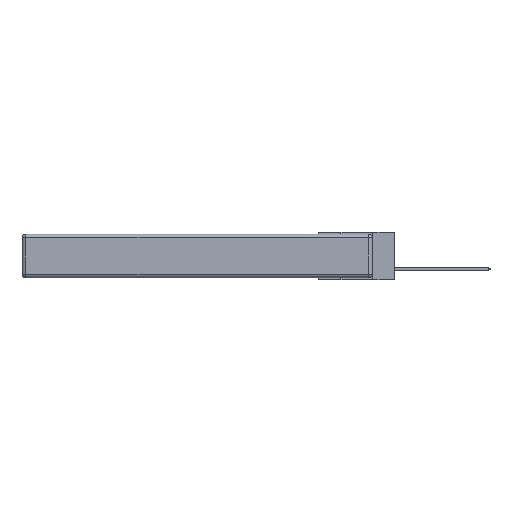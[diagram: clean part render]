
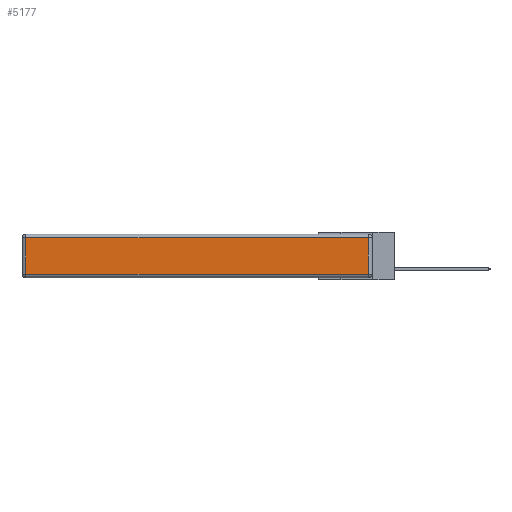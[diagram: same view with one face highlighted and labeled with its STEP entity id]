
A CAD part, left-side view. The second image highlights one B-rep face of the part: STEP entity #5177.
In plain terms, the highlighted planar face has unit normal (-1, 0, 0).
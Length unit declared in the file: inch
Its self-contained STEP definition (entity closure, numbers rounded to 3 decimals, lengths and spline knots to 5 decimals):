
#218 = CARTESIAN_POINT ( 'NONE',  ( 0., 0., -0.313 ) ) ;
#310 = DIRECTION ( 'NONE',  ( 0., -1., 0. ) ) ;
#544 = DIRECTION ( 'NONE',  ( 0., 0., -1. ) ) ;
#930 = DIRECTION ( 'NONE',  ( 0., 0., 1. ) ) ;
#1466 = AXIS2_PLACEMENT_3D ( 'NONE', #8720, #6859, #4696 ) ;
#1596 = CARTESIAN_POINT ( 'NONE',  ( 0., 2.72, -0.343 ) ) ;
#1698 = LINE ( 'NONE', #3407, #12621 ) ;
#1766 = ORIENTED_EDGE ( 'NONE', *, *, #7449, .T. ) ;
#2106 = VECTOR ( 'NONE', #544, 39.37008 ) ;
#3407 = CARTESIAN_POINT ( 'NONE',  ( 0., 2.75, -0.03 ) ) ;
#4056 = CARTESIAN_POINT ( 'NONE',  ( 0., 0.03, -0.343 ) ) ;
#4112 = LINE ( 'NONE', #4056, #12896 ) ;
#4338 = VERTEX_POINT ( 'NONE', #11264 ) ;
#4463 = ORIENTED_EDGE ( 'NONE', *, *, #11838, .T. ) ;
#4696 = DIRECTION ( 'NONE',  ( 0., 0., 1. ) ) ;
#4885 = VECTOR ( 'NONE', #310, 39.37008 ) ;
#5177 = ADVANCED_FACE ( 'NONE', ( #6686 ), #7773, .T. ) ;
#5509 = ORIENTED_EDGE ( 'NONE', *, *, #12189, .T. ) ;
#5914 = CARTESIAN_POINT ( 'NONE',  ( 0., 2.72, -0.03 ) ) ;
#5949 = CARTESIAN_POINT ( 'NONE',  ( 0., 0.03, -0.03 ) ) ;
#6259 = LINE ( 'NONE', #1596, #2106 ) ;
#6686 = FACE_OUTER_BOUND ( 'NONE', #10412, .T. ) ;
#6859 = DIRECTION ( 'NONE',  ( -1., 0., 0. ) ) ;
#7120 = VERTEX_POINT ( 'NONE', #5914 ) ;
#7449 = EDGE_CURVE ( 'NONE', #12579, #7120, #1698, .T. ) ;
#7675 = LINE ( 'NONE', #218, #4885 ) ;
#7773 = PLANE ( 'NONE',  #1466 ) ;
#8720 = CARTESIAN_POINT ( 'NONE',  ( 0., 0., -0.343 ) ) ;
#9785 = CARTESIAN_POINT ( 'NONE',  ( 0., 0.03, -0.313 ) ) ;
#10412 = EDGE_LOOP ( 'NONE', ( #13612, #4463, #1766, #5509 ) ) ;
#10650 = DIRECTION ( 'NONE',  ( 0., 1., 0. ) ) ;
#11264 = CARTESIAN_POINT ( 'NONE',  ( 0., 2.72, -0.313 ) ) ;
#11361 = VERTEX_POINT ( 'NONE', #9785 ) ;
#11838 = EDGE_CURVE ( 'NONE', #11361, #12579, #4112, .T. ) ;
#12189 = EDGE_CURVE ( 'NONE', #7120, #4338, #6259, .T. ) ;
#12579 = VERTEX_POINT ( 'NONE', #5949 ) ;
#12621 = VECTOR ( 'NONE', #10650, 39.37008 ) ;
#12896 = VECTOR ( 'NONE', #930, 39.37008 ) ;
#13550 = EDGE_CURVE ( 'NONE', #4338, #11361, #7675, .T. ) ;
#13612 = ORIENTED_EDGE ( 'NONE', *, *, #13550, .T. ) ;
